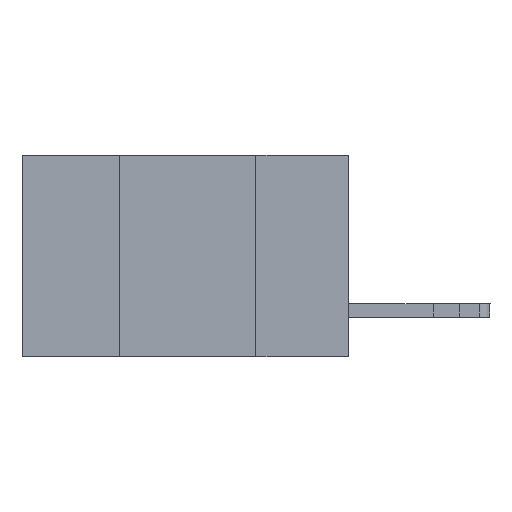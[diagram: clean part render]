
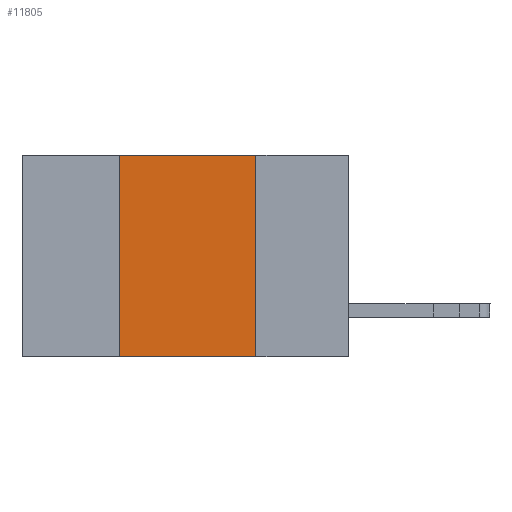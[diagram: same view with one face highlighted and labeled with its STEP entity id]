
A CAD part, left-side view. The second image highlights one B-rep face of the part: STEP entity #11805.
In plain terms, the highlighted planar face has unit normal (-1, 0, 0).
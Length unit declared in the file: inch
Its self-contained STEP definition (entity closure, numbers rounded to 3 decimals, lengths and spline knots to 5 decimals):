
#780 = LINE ( 'NONE', #6910, #4097 ) ;
#852 = ORIENTED_EDGE ( 'NONE', *, *, #13532, .T. ) ;
#1484 = EDGE_LOOP ( 'NONE', ( #8557, #2375, #10944, #852 ) ) ;
#1508 = PLANE ( 'NONE',  #5145 ) ;
#1548 = VERTEX_POINT ( 'NONE', #7316 ) ;
#2375 = ORIENTED_EDGE ( 'NONE', *, *, #12452, .F. ) ;
#2756 = EDGE_CURVE ( 'NONE', #10978, #4086, #5711, .T. ) ;
#2779 = DIRECTION ( 'NONE',  ( 0., -1., 0. ) ) ;
#2858 = VECTOR ( 'NONE', #12745, 39.37008 ) ;
#3551 = DIRECTION ( 'NONE',  ( 0., -1., 0. ) ) ;
#3699 = CARTESIAN_POINT ( 'NONE',  ( 0., 0.17, -0.37 ) ) ;
#4086 = VERTEX_POINT ( 'NONE', #3699 ) ;
#4097 = VECTOR ( 'NONE', #2779, 39.37008 ) ;
#5106 = CARTESIAN_POINT ( 'NONE',  ( 0., 0.17, -0.37 ) ) ;
#5112 = VECTOR ( 'NONE', #3551, 39.37008 ) ;
#5142 = VECTOR ( 'NONE', #5703, 39.37008 ) ;
#5145 = AXIS2_PLACEMENT_3D ( 'NONE', #13084, #7761, #8813 ) ;
#5622 = CARTESIAN_POINT ( 'NONE',  ( 0., 0.6, -0.37 ) ) ;
#5703 = DIRECTION ( 'NONE',  ( 0., 0., 1. ) ) ;
#5711 = LINE ( 'NONE', #5106, #2858 ) ;
#6069 = EDGE_CURVE ( 'NONE', #9019, #1548, #10228, .T. ) ;
#6276 = FACE_OUTER_BOUND ( 'NONE', #1484, .T. ) ;
#6910 = CARTESIAN_POINT ( 'NONE',  ( 0., 0.6, 0. ) ) ;
#7316 = CARTESIAN_POINT ( 'NONE',  ( 0., 0.42, 0. ) ) ;
#7761 = DIRECTION ( 'NONE',  ( 1., 0., 0. ) ) ;
#8385 = LINE ( 'NONE', #5622, #5112 ) ;
#8557 = ORIENTED_EDGE ( 'NONE', *, *, #2756, .F. ) ;
#8791 = CARTESIAN_POINT ( 'NONE',  ( 0., 0.17, 0. ) ) ;
#8813 = DIRECTION ( 'NONE',  ( 0., 0., -1. ) ) ;
#9019 = VERTEX_POINT ( 'NONE', #10802 ) ;
#9907 = CARTESIAN_POINT ( 'NONE',  ( 0., 0.42, -0.37 ) ) ;
#10228 = LINE ( 'NONE', #9907, #5142 ) ;
#10802 = CARTESIAN_POINT ( 'NONE',  ( 0., 0.42, -0.37 ) ) ;
#10944 = ORIENTED_EDGE ( 'NONE', *, *, #6069, .F. ) ;
#10978 = VERTEX_POINT ( 'NONE', #8791 ) ;
#11805 = ADVANCED_FACE ( 'NONE', ( #6276 ), #1508, .F. ) ;
#12452 = EDGE_CURVE ( 'NONE', #1548, #10978, #780, .T. ) ;
#12745 = DIRECTION ( 'NONE',  ( 0., 0., -1. ) ) ;
#13084 = CARTESIAN_POINT ( 'NONE',  ( 0., 0.6, 0. ) ) ;
#13532 = EDGE_CURVE ( 'NONE', #9019, #4086, #8385, .T. ) ;
